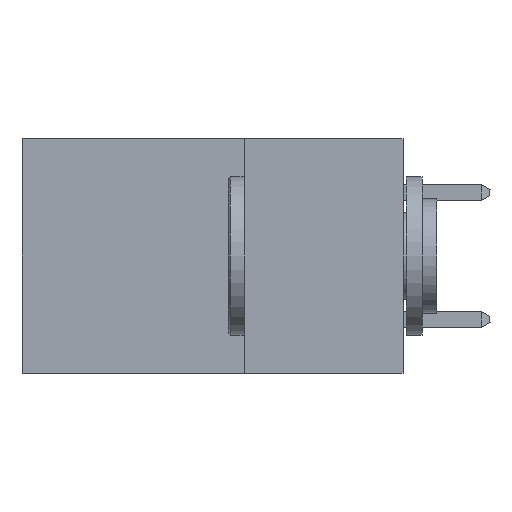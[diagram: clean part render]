
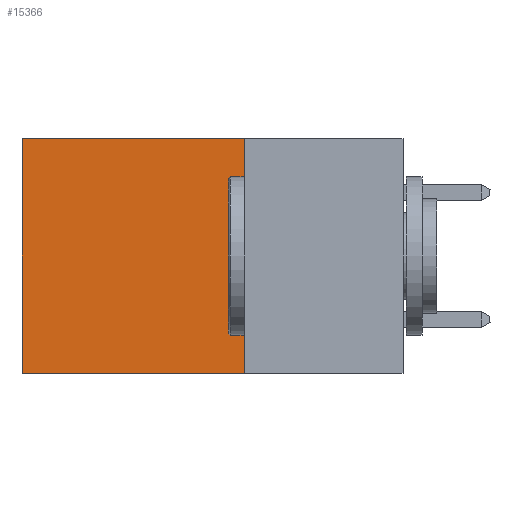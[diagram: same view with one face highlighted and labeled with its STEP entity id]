
A CAD part, left-side view. The second image highlights one B-rep face of the part: STEP entity #15366.
In plain terms, the highlighted planar face has unit normal (-1, 0, 0).
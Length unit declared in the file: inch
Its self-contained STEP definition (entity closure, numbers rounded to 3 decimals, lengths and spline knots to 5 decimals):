
#1553 = VERTEX_POINT ( 'NONE', #10023 ) ;
#2936 = AXIS2_PLACEMENT_3D ( 'NONE', #33017, #27475, #15455 ) ;
#5588 = DIRECTION ( 'NONE',  ( 0., 1., 0. ) ) ;
#8139 = VERTEX_POINT ( 'NONE', #26757 ) ;
#8395 = CARTESIAN_POINT ( 'NONE',  ( 0.2875, 0.25, 0. ) ) ;
#9483 = EDGE_CURVE ( 'NONE', #1553, #32361, #20653, .T. ) ;
#9895 = LINE ( 'NONE', #22291, #28890 ) ;
#10023 = CARTESIAN_POINT ( 'NONE',  ( 0.2875, 0.25, -0.37 ) ) ;
#10157 = ORIENTED_EDGE ( 'NONE', *, *, #31674, .T. ) ;
#11496 = VERTEX_POINT ( 'NONE', #19374 ) ;
#14412 = VECTOR ( 'NONE', #5588, 39.37008 ) ;
#14631 = EDGE_CURVE ( 'NONE', #8139, #1553, #31597, .T. ) ;
#15366 = ADVANCED_FACE ( 'NONE', ( #22030 ), #18735, .F. ) ;
#15455 = DIRECTION ( 'NONE',  ( 0., 0., -1. ) ) ;
#15685 = ORIENTED_EDGE ( 'NONE', *, *, #9483, .F. ) ;
#18336 = VECTOR ( 'NONE', #34090, 39.37008 ) ;
#18735 = PLANE ( 'NONE',  #2936 ) ;
#19374 = CARTESIAN_POINT ( 'NONE',  ( 0.2875, 0.6, 0. ) ) ;
#20653 = LINE ( 'NONE', #25245, #18336 ) ;
#22030 = FACE_OUTER_BOUND ( 'NONE', #26559, .T. ) ;
#22291 = CARTESIAN_POINT ( 'NONE',  ( 0.2875, 0.6, 0. ) ) ;
#24258 = EDGE_CURVE ( 'NONE', #8139, #11496, #34772, .T. ) ;
#24375 = DIRECTION ( 'NONE',  ( 0., 0., -1. ) ) ;
#25245 = CARTESIAN_POINT ( 'NONE',  ( 0.2875, 0.25, -0.37 ) ) ;
#25266 = VECTOR ( 'NONE', #24375, 39.37008 ) ;
#26559 = EDGE_LOOP ( 'NONE', ( #10157, #15685, #34717, #35023 ) ) ;
#26757 = CARTESIAN_POINT ( 'NONE',  ( 0.2875, 0.25, 0. ) ) ;
#27475 = DIRECTION ( 'NONE',  ( 1., 0., 0. ) ) ;
#28890 = VECTOR ( 'NONE', #36973, 39.37008 ) ;
#30060 = CARTESIAN_POINT ( 'NONE',  ( 0.2875, 0.25, 0. ) ) ;
#30842 = CARTESIAN_POINT ( 'NONE',  ( 0.2875, 0.6, -0.37 ) ) ;
#31597 = LINE ( 'NONE', #30060, #25266 ) ;
#31674 = EDGE_CURVE ( 'NONE', #11496, #32361, #9895, .T. ) ;
#32361 = VERTEX_POINT ( 'NONE', #30842 ) ;
#33017 = CARTESIAN_POINT ( 'NONE',  ( 0.2875, 0.25, 0. ) ) ;
#34090 = DIRECTION ( 'NONE',  ( 0., 1., 0. ) ) ;
#34717 = ORIENTED_EDGE ( 'NONE', *, *, #14631, .F. ) ;
#34772 = LINE ( 'NONE', #8395, #14412 ) ;
#35023 = ORIENTED_EDGE ( 'NONE', *, *, #24258, .T. ) ;
#36973 = DIRECTION ( 'NONE',  ( 0., 0., -1. ) ) ;
